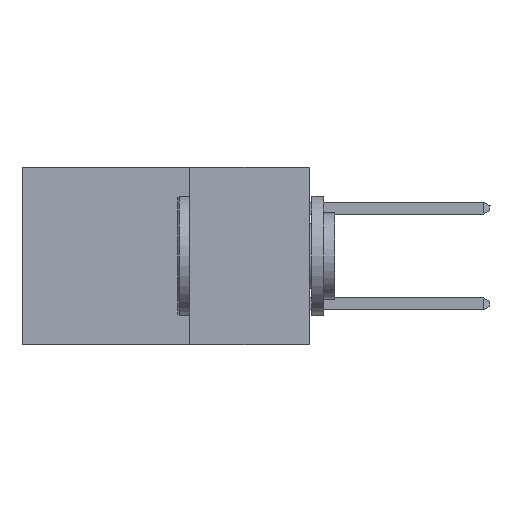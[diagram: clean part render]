
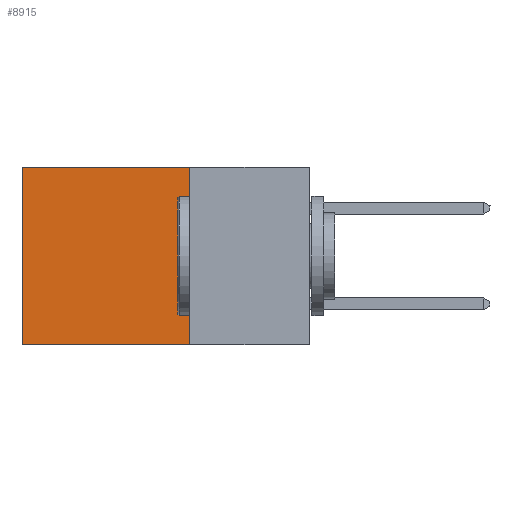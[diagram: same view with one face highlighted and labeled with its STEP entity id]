
A CAD part, left-side view. The second image highlights one B-rep face of the part: STEP entity #8915.
In plain terms, the highlighted planar face has unit normal (-1, 0, 0).
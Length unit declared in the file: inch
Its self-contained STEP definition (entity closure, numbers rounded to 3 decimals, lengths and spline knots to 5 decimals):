
#753 = VERTEX_POINT ( 'NONE', #5401 ) ;
#928 = DIRECTION ( 'NONE',  ( 0., 1., 0. ) ) ;
#5304 = VECTOR ( 'NONE', #928, 39.37008 ) ;
#5401 = CARTESIAN_POINT ( 'NONE',  ( 0.2875, 0.25, 0. ) ) ;
#5681 = VECTOR ( 'NONE', #29691, 39.37008 ) ;
#6269 = LINE ( 'NONE', #25108, #5304 ) ;
#6607 = ORIENTED_EDGE ( 'NONE', *, *, #36872, .F. ) ;
#8915 = ADVANCED_FACE ( 'NONE', ( #32181 ), #16604, .F. ) ;
#10401 = VERTEX_POINT ( 'NONE', #17646 ) ;
#10900 = CARTESIAN_POINT ( 'NONE',  ( 0.2875, 0.25, 0. ) ) ;
#12480 = CARTESIAN_POINT ( 'NONE',  ( 0.2875, 0.25, -0.37 ) ) ;
#13660 = ORIENTED_EDGE ( 'NONE', *, *, #30565, .T. ) ;
#13672 = AXIS2_PLACEMENT_3D ( 'NONE', #10900, #16863, #25634 ) ;
#15525 = DIRECTION ( 'NONE',  ( 0., 1., 0. ) ) ;
#16453 = EDGE_CURVE ( 'NONE', #23150, #10401, #29060, .T. ) ;
#16604 = PLANE ( 'NONE',  #13672 ) ;
#16863 = DIRECTION ( 'NONE',  ( 1., 0., 0. ) ) ;
#17646 = CARTESIAN_POINT ( 'NONE',  ( 0.2875, 0.6, -0.37 ) ) ;
#17685 = VECTOR ( 'NONE', #30019, 39.37008 ) ;
#18836 = ORIENTED_EDGE ( 'NONE', *, *, #16453, .T. ) ;
#20320 = CARTESIAN_POINT ( 'NONE',  ( 0.2875, 0.6, 0. ) ) ;
#21171 = CARTESIAN_POINT ( 'NONE',  ( 0.2875, 0.25, 0. ) ) ;
#22492 = CARTESIAN_POINT ( 'NONE',  ( 0.2875, 0.25, -0.37 ) ) ;
#23150 = VERTEX_POINT ( 'NONE', #20320 ) ;
#24806 = LINE ( 'NONE', #21171, #17685 ) ;
#25108 = CARTESIAN_POINT ( 'NONE',  ( 0.2875, 0.25, 0. ) ) ;
#25634 = DIRECTION ( 'NONE',  ( 0., 0., -1. ) ) ;
#29060 = LINE ( 'NONE', #35547, #5681 ) ;
#29691 = DIRECTION ( 'NONE',  ( 0., 0., -1. ) ) ;
#29861 = ORIENTED_EDGE ( 'NONE', *, *, #31123, .F. ) ;
#30019 = DIRECTION ( 'NONE',  ( 0., 0., -1. ) ) ;
#30565 = EDGE_CURVE ( 'NONE', #753, #23150, #6269, .T. ) ;
#31123 = EDGE_CURVE ( 'NONE', #38981, #10401, #36744, .T. ) ;
#32181 = FACE_OUTER_BOUND ( 'NONE', #36038, .T. ) ;
#33868 = VECTOR ( 'NONE', #15525, 39.37008 ) ;
#35547 = CARTESIAN_POINT ( 'NONE',  ( 0.2875, 0.6, 0. ) ) ;
#36038 = EDGE_LOOP ( 'NONE', ( #18836, #29861, #6607, #13660 ) ) ;
#36744 = LINE ( 'NONE', #12480, #33868 ) ;
#36872 = EDGE_CURVE ( 'NONE', #753, #38981, #24806, .T. ) ;
#38981 = VERTEX_POINT ( 'NONE', #22492 ) ;
